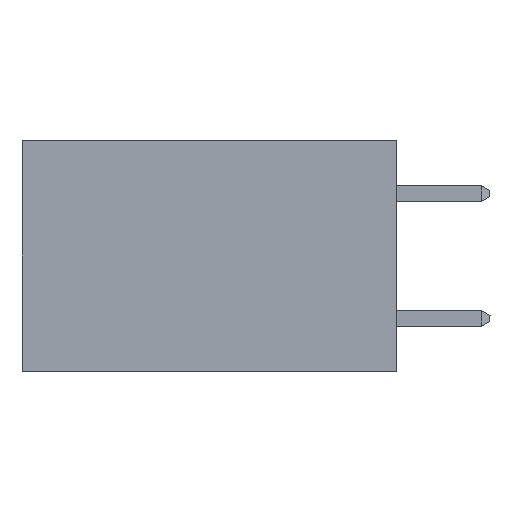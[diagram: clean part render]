
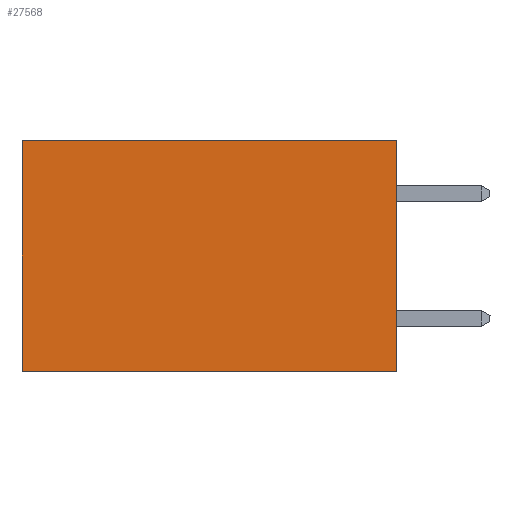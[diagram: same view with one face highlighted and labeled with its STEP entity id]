
A CAD part, left-side view. The second image highlights one B-rep face of the part: STEP entity #27568.
In plain terms, the highlighted planar face has unit normal (-1, 0, 0).
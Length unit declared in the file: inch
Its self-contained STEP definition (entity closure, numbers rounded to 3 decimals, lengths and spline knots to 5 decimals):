
#145 = DIRECTION ( 'NONE',  ( 0., 0., -1. ) ) ;
#437 = EDGE_LOOP ( 'NONE', ( #16399, #22728, #774, #30715 ) ) ;
#684 = CARTESIAN_POINT ( 'NONE',  ( 0.298, 0., 0. ) ) ;
#774 = ORIENTED_EDGE ( 'NONE', *, *, #10009, .F. ) ;
#2954 = FACE_OUTER_BOUND ( 'NONE', #437, .T. ) ;
#3063 = CARTESIAN_POINT ( 'NONE',  ( 0.298, 0., -0.37 ) ) ;
#4443 = VERTEX_POINT ( 'NONE', #684 ) ;
#7045 = CARTESIAN_POINT ( 'NONE',  ( 0.298, 0., 0. ) ) ;
#7126 = VERTEX_POINT ( 'NONE', #7849 ) ;
#7796 = LINE ( 'NONE', #13808, #26850 ) ;
#7849 = CARTESIAN_POINT ( 'NONE',  ( 0.298, 0.6, 0. ) ) ;
#10009 = EDGE_CURVE ( 'NONE', #4443, #25112, #12787, .T. ) ;
#10915 = LINE ( 'NONE', #3063, #22598 ) ;
#10951 = EDGE_CURVE ( 'NONE', #7126, #27521, #11854, .T. ) ;
#11854 = LINE ( 'NONE', #12297, #12250 ) ;
#12250 = VECTOR ( 'NONE', #26781, 39.37008 ) ;
#12297 = CARTESIAN_POINT ( 'NONE',  ( 0.298, 0.6, 0. ) ) ;
#12787 = LINE ( 'NONE', #27848, #30723 ) ;
#13808 = CARTESIAN_POINT ( 'NONE',  ( 0.298, 0., 0. ) ) ;
#13815 = EDGE_CURVE ( 'NONE', #25112, #27521, #10915, .T. ) ;
#16399 = ORIENTED_EDGE ( 'NONE', *, *, #10951, .T. ) ;
#18417 = CARTESIAN_POINT ( 'NONE',  ( 0.298, 0., -0.37 ) ) ;
#19314 = DIRECTION ( 'NONE',  ( 0., 0., -1. ) ) ;
#20839 = AXIS2_PLACEMENT_3D ( 'NONE', #7045, #26729, #19314 ) ;
#20911 = DIRECTION ( 'NONE',  ( 0., 1., 0. ) ) ;
#21938 = PLANE ( 'NONE',  #20839 ) ;
#22598 = VECTOR ( 'NONE', #20911, 39.37008 ) ;
#22728 = ORIENTED_EDGE ( 'NONE', *, *, #13815, .F. ) ;
#25112 = VERTEX_POINT ( 'NONE', #18417 ) ;
#26729 = DIRECTION ( 'NONE',  ( 1., 0., 0. ) ) ;
#26781 = DIRECTION ( 'NONE',  ( 0., 0., -1. ) ) ;
#26850 = VECTOR ( 'NONE', #28535, 39.37008 ) ;
#27521 = VERTEX_POINT ( 'NONE', #29218 ) ;
#27568 = ADVANCED_FACE ( 'NONE', ( #2954 ), #21938, .F. ) ;
#27848 = CARTESIAN_POINT ( 'NONE',  ( 0.298, 0., 0. ) ) ;
#28535 = DIRECTION ( 'NONE',  ( 0., 1., 0. ) ) ;
#29218 = CARTESIAN_POINT ( 'NONE',  ( 0.298, 0.6, -0.37 ) ) ;
#30715 = ORIENTED_EDGE ( 'NONE', *, *, #30975, .T. ) ;
#30723 = VECTOR ( 'NONE', #145, 39.37008 ) ;
#30975 = EDGE_CURVE ( 'NONE', #4443, #7126, #7796, .T. ) ;
